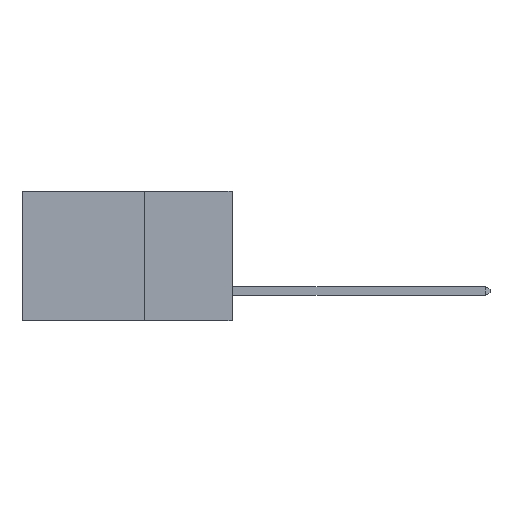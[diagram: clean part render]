
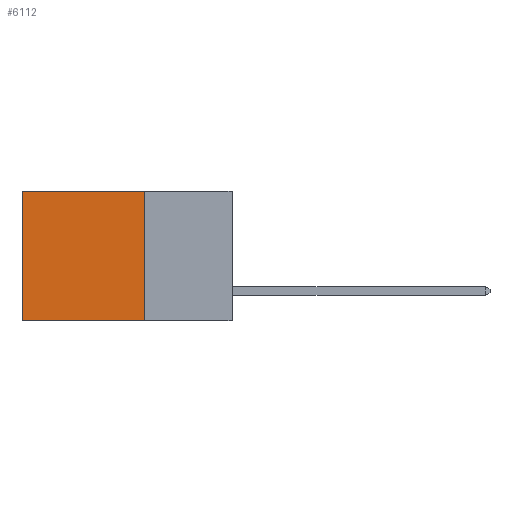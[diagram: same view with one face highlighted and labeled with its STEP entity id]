
A CAD part, left-side view. The second image highlights one B-rep face of the part: STEP entity #6112.
In plain terms, the highlighted planar face has unit normal (-1, 0, 0).
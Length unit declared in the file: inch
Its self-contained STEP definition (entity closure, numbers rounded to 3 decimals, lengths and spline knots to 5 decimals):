
#227 = DIRECTION ( 'NONE',  ( 0., 0., -1. ) ) ;
#304 = EDGE_CURVE ( 'NONE', #1603, #10616, #4060, .T. ) ;
#737 = EDGE_CURVE ( 'NONE', #4254, #10257, #4576, .T. ) ;
#890 = DIRECTION ( 'NONE',  ( 0., 0., -1. ) ) ;
#1120 = LINE ( 'NONE', #5543, #11908 ) ;
#1492 = ORIENTED_EDGE ( 'NONE', *, *, #4402, .F. ) ;
#1603 = VERTEX_POINT ( 'NONE', #3417 ) ;
#1810 = CARTESIAN_POINT ( 'NONE',  ( 0.2875, 0.25, -0.37 ) ) ;
#1823 = CARTESIAN_POINT ( 'NONE',  ( 0.2875, 0.25, 0. ) ) ;
#2845 = ORIENTED_EDGE ( 'NONE', *, *, #5457, .T. ) ;
#2941 = DIRECTION ( 'NONE',  ( 0., 1., 0. ) ) ;
#3212 = AXIS2_PLACEMENT_3D ( 'NONE', #1823, #12263, #6119 ) ;
#3231 = CARTESIAN_POINT ( 'NONE',  ( 0.2875, 0.6, 0. ) ) ;
#3417 = CARTESIAN_POINT ( 'NONE',  ( 0.2875, 0.25, 0. ) ) ;
#3953 = VECTOR ( 'NONE', #2941, 39.37008 ) ;
#4060 = LINE ( 'NONE', #4429, #9286 ) ;
#4254 = VERTEX_POINT ( 'NONE', #3231 ) ;
#4402 = EDGE_CURVE ( 'NONE', #10616, #10257, #1120, .T. ) ;
#4429 = CARTESIAN_POINT ( 'NONE',  ( 0.2875, 0.25, 0. ) ) ;
#4576 = LINE ( 'NONE', #5163, #12144 ) ;
#5078 = PLANE ( 'NONE',  #3212 ) ;
#5163 = CARTESIAN_POINT ( 'NONE',  ( 0.2875, 0.6, 0. ) ) ;
#5457 = EDGE_CURVE ( 'NONE', #1603, #4254, #11882, .T. ) ;
#5543 = CARTESIAN_POINT ( 'NONE',  ( 0.2875, 0.25, -0.37 ) ) ;
#6112 = ADVANCED_FACE ( 'NONE', ( #6901 ), #5078, .F. ) ;
#6119 = DIRECTION ( 'NONE',  ( 0., 0., -1. ) ) ;
#6656 = EDGE_LOOP ( 'NONE', ( #13143, #1492, #12530, #2845 ) ) ;
#6901 = FACE_OUTER_BOUND ( 'NONE', #6656, .T. ) ;
#7623 = DIRECTION ( 'NONE',  ( 0., 1., 0. ) ) ;
#9286 = VECTOR ( 'NONE', #227, 39.37008 ) ;
#10257 = VERTEX_POINT ( 'NONE', #12818 ) ;
#10616 = VERTEX_POINT ( 'NONE', #1810 ) ;
#11240 = CARTESIAN_POINT ( 'NONE',  ( 0.2875, 0.25, 0. ) ) ;
#11882 = LINE ( 'NONE', #11240, #3953 ) ;
#11908 = VECTOR ( 'NONE', #7623, 39.37008 ) ;
#12144 = VECTOR ( 'NONE', #890, 39.37008 ) ;
#12263 = DIRECTION ( 'NONE',  ( 1., 0., 0. ) ) ;
#12530 = ORIENTED_EDGE ( 'NONE', *, *, #304, .F. ) ;
#12818 = CARTESIAN_POINT ( 'NONE',  ( 0.2875, 0.6, -0.37 ) ) ;
#13143 = ORIENTED_EDGE ( 'NONE', *, *, #737, .T. ) ;
